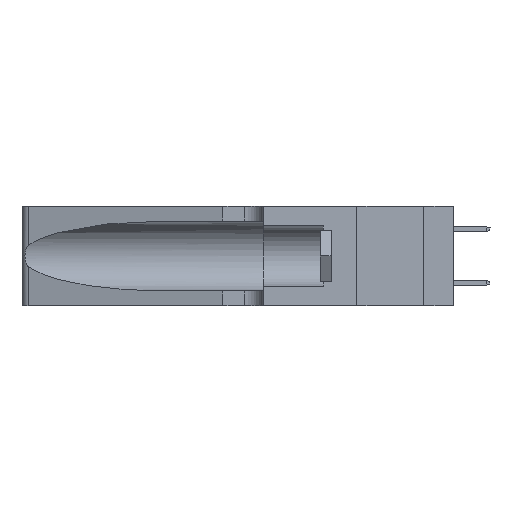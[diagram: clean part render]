
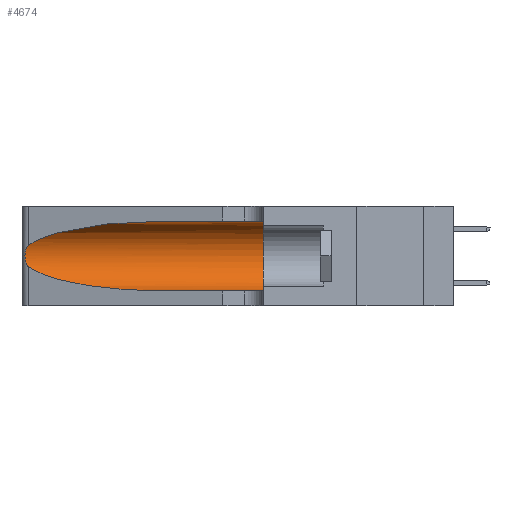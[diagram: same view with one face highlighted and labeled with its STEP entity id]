
A CAD part, left-side view. The second image highlights one B-rep face of the part: STEP entity #4674.
In plain terms, the highlighted cylindrical face has radius 3.308 mm (diameter 6.617 mm), a partial arc.
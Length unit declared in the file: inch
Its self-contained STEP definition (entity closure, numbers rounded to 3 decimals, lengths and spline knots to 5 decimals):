
#782 = EDGE_CURVE ( 'NONE', #13216, #13734, #2381, .T. ) ;
#1261 = EDGE_CURVE ( 'NONE', #18757, #6948, #6478, .T. ) ;
#1505 = CARTESIAN_POINT ( 'NONE',  ( 0.25639, 1.23184, 0.21858 ) ) ;
#2043 = EDGE_CURVE ( 'NONE', #6948, #9261, #18619, .T. ) ;
#2266 = VECTOR ( 'NONE', #4186, 39.37008 ) ;
#2358 = EDGE_CURVE ( 'NONE', #13734, #9261, #14177, .T. ) ;
#2381 =( BOUNDED_CURVE ( )  B_SPLINE_CURVE ( 3, ( #3116, #10709, #4769, #7696 ),
 .UNSPECIFIED., .F., .F. ) 
 B_SPLINE_CURVE_WITH_KNOTS ( ( 4, 4 ),
 ( 3.44316, 4.71239 ),
 .UNSPECIFIED. ) 
 CURVE ( )  GEOMETRIC_REPRESENTATION_ITEM ( )  RATIONAL_B_SPLINE_CURVE ( ( 1., 0.87, 0.87, 1. ) ) 
 REPRESENTATION_ITEM ( '' )  );
#2388 = DIRECTION ( 'NONE',  ( 0., 0., -1. ) ) ;
#3116 = CARTESIAN_POINT ( 'NONE',  ( 0.25487, 1.22718, 0.14631 ) ) ;
#3258 = CARTESIAN_POINT ( 'NONE',  ( 0.25639, 1.23186, 0.15144 ) ) ;
#3273 = VECTOR ( 'NONE', #16708, 39.37008 ) ;
#4037 = CYLINDRICAL_SURFACE ( 'NONE', #10540, 0.13025 ) ;
#4055 = CARTESIAN_POINT ( 'NONE',  ( 0.26018, 1.23835, 0.19895 ) ) ;
#4186 = DIRECTION ( 'NONE',  ( 0., -1., 0. ) ) ;
#4299 = DIRECTION ( 'NONE',  ( 0., 1., 0. ) ) ;
#4398 = DIRECTION ( 'NONE',  ( 0., 0., 1. ) ) ;
#4674 = ADVANCED_FACE ( 'NONE', ( #9965 ), #4037, .F. ) ;
#4769 = CARTESIAN_POINT ( 'NONE',  ( 0.18966, 0.96281, 0.05475 ) ) ;
#5387 = CARTESIAN_POINT ( 'NONE',  ( 0.1305, 1.61858, 0.185 ) ) ;
#5508 = CARTESIAN_POINT ( 'NONE',  ( 0.25787, 1.23484, 0.2124 ) ) ;
#6478 = LINE ( 'NONE', #18449, #3273 ) ;
#6693 = VERTEX_POINT ( 'NONE', #7790 ) ;
#6948 = VERTEX_POINT ( 'NONE', #11658 ) ;
#7315 = CARTESIAN_POINT ( 'NONE',  ( 0.1305, 0.35, 0.185 ) ) ;
#7440 = CARTESIAN_POINT ( 'NONE',  ( 0.25555, 1.22993, 0.14849 ) ) ;
#7641 = CARTESIAN_POINT ( 'NONE',  ( 0.26017, 1.23833, 0.17102 ) ) ;
#7696 = CARTESIAN_POINT ( 'NONE',  ( 0.1305, 0.72297, 0.05475 ) ) ;
#7790 = CARTESIAN_POINT ( 'NONE',  ( 0.25487, 1.22718, 0.22369 ) ) ;
#9169 = EDGE_LOOP ( 'NONE', ( #18243, #12113, #10695, #18408, #14321, #10588 ) ) ;
#9261 = VERTEX_POINT ( 'NONE', #15045 ) ;
#9288 = CARTESIAN_POINT ( 'NONE',  ( 0.26075, 1.23896, 0.178 ) ) ;
#9386 = CARTESIAN_POINT ( 'NONE',  ( 0.25856, 1.23593, 0.16098 ) ) ;
#9965 = FACE_OUTER_BOUND ( 'NONE', #9169, .T. ) ;
#10181 = CARTESIAN_POINT ( 'NONE',  ( 0.25487, 1.22718, 0.22369 ) ) ;
#10486 = B_SPLINE_CURVE_WITH_KNOTS ( 'NONE', 3,
 ( #10181, #18738, #1505, #5508, #11432, #4055, #13729, #9288, #7641, #9386, #10750, #3258, #7440, #16504 ),
 .UNSPECIFIED., .F., .F.,
 ( 4, 2, 2, 2, 2, 2, 4 ),
 ( 0., 0.00027, 0.00053, 0.00107, 0.0016, 0.00187, 0.00214 ),
 .UNSPECIFIED. ) ;
#10540 = AXIS2_PLACEMENT_3D ( 'NONE', #5387, #16045, #2388 ) ;
#10588 = ORIENTED_EDGE ( 'NONE', *, *, #1261, .F. ) ;
#10695 = ORIENTED_EDGE ( 'NONE', *, *, #782, .T. ) ;
#10709 = CARTESIAN_POINT ( 'NONE',  ( 0.2373, 1.15595, 0.08982 ) ) ;
#10750 = CARTESIAN_POINT ( 'NONE',  ( 0.25789, 1.23486, 0.15765 ) ) ;
#10877 = CARTESIAN_POINT ( 'NONE',  ( 0.1305, 0.72297, 0.05475 ) ) ;
#11408 = CARTESIAN_POINT ( 'NONE',  ( 0.1305, 0.72297, 0.31525 ) ) ;
#11432 = CARTESIAN_POINT ( 'NONE',  ( 0.25854, 1.2359, 0.20912 ) ) ;
#11658 = CARTESIAN_POINT ( 'NONE',  ( 0.1305, 0.35, 0.31525 ) ) ;
#12113 = ORIENTED_EDGE ( 'NONE', *, *, #15979, .T. ) ;
#12812 = CARTESIAN_POINT ( 'NONE',  ( 0.1305, 1.61858, 0.05475 ) ) ;
#13216 = VERTEX_POINT ( 'NONE', #19082 ) ;
#13729 = CARTESIAN_POINT ( 'NONE',  ( 0.26075, 1.23896, 0.19203 ) ) ;
#13734 = VERTEX_POINT ( 'NONE', #10877 ) ;
#14177 = LINE ( 'NONE', #12812, #2266 ) ;
#14321 = ORIENTED_EDGE ( 'NONE', *, *, #2043, .F. ) ;
#15045 = CARTESIAN_POINT ( 'NONE',  ( 0.1305, 0.35, 0.05475 ) ) ;
#15756 = CARTESIAN_POINT ( 'NONE',  ( 0.2373, 1.15595, 0.28018 ) ) ;
#15979 = EDGE_CURVE ( 'NONE', #6693, #13216, #10486, .T. ) ;
#16045 = DIRECTION ( 'NONE',  ( 0., -1., 0. ) ) ;
#16311 = EDGE_CURVE ( 'NONE', #18757, #6693, #16949, .T. ) ;
#16504 = CARTESIAN_POINT ( 'NONE',  ( 0.25487, 1.22718, 0.14631 ) ) ;
#16708 = DIRECTION ( 'NONE',  ( 0., -1., 0. ) ) ;
#16785 = AXIS2_PLACEMENT_3D ( 'NONE', #7315, #4299, #4398 ) ;
#16949 =( BOUNDED_CURVE ( )  B_SPLINE_CURVE ( 3, ( #11408, #17357, #15756, #17263 ),
 .UNSPECIFIED., .F., .F. ) 
 B_SPLINE_CURVE_WITH_KNOTS ( ( 4, 4 ),
 ( 1.5708, 2.84003 ),
 .UNSPECIFIED. ) 
 CURVE ( )  GEOMETRIC_REPRESENTATION_ITEM ( )  RATIONAL_B_SPLINE_CURVE ( ( 1., 0.87, 0.87, 1. ) ) 
 REPRESENTATION_ITEM ( '' )  );
#17263 = CARTESIAN_POINT ( 'NONE',  ( 0.25487, 1.22718, 0.22369 ) ) ;
#17357 = CARTESIAN_POINT ( 'NONE',  ( 0.18966, 0.96281, 0.31525 ) ) ;
#17407 = CARTESIAN_POINT ( 'NONE',  ( 0.1305, 0.72297, 0.31525 ) ) ;
#18243 = ORIENTED_EDGE ( 'NONE', *, *, #16311, .T. ) ;
#18408 = ORIENTED_EDGE ( 'NONE', *, *, #2358, .T. ) ;
#18449 = CARTESIAN_POINT ( 'NONE',  ( 0.1305, 1.61858, 0.31525 ) ) ;
#18619 = CIRCLE ( 'NONE', #16785, 0.13025 ) ;
#18738 = CARTESIAN_POINT ( 'NONE',  ( 0.25555, 1.22994, 0.2215 ) ) ;
#18757 = VERTEX_POINT ( 'NONE', #17407 ) ;
#19082 = CARTESIAN_POINT ( 'NONE',  ( 0.25487, 1.22718, 0.14631 ) ) ;
